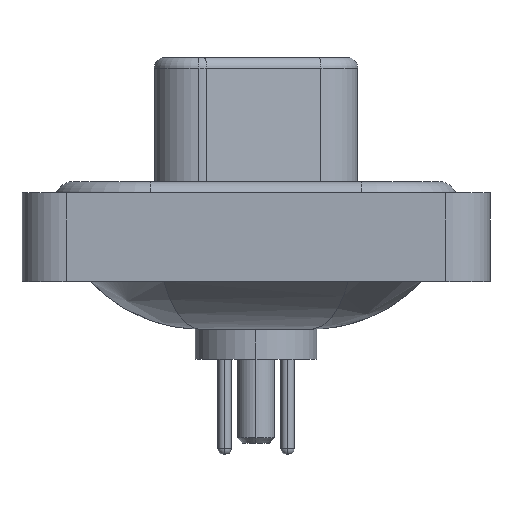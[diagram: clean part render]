
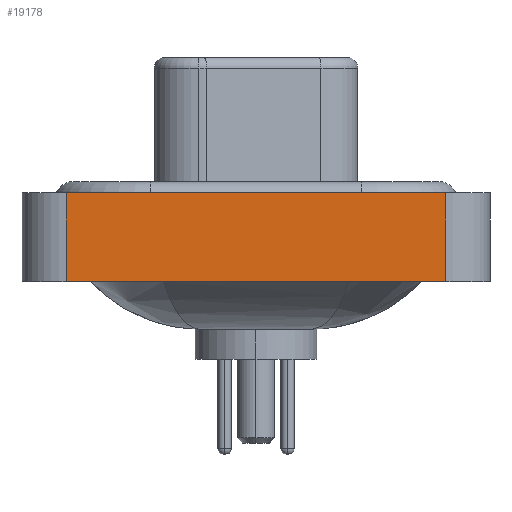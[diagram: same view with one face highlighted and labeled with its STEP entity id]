
A CAD part, left-side view. The second image highlights one B-rep face of the part: STEP entity #19178.
In plain terms, the highlighted planar face has unit normal (-1, 0, 0).
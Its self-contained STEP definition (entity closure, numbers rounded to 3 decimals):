
#711 = EDGE_LOOP ( 'NONE', ( #2815, #13599, #16392, #7864 ) ) ;
#886 = VECTOR ( 'NONE', #18986, 1000. ) ;
#1263 = DIRECTION ( 'NONE',  ( 0., 0., 1. ) ) ;
#2015 = VERTEX_POINT ( 'NONE', #18123 ) ;
#2815 = ORIENTED_EDGE ( 'NONE', *, *, #9867, .T. ) ;
#3252 = CARTESIAN_POINT ( 'NONE',  ( -7.3, -8.55, -3.6 ) ) ;
#3781 = VECTOR ( 'NONE', #5715, 1000. ) ;
#4097 = CARTESIAN_POINT ( 'NONE',  ( -7.3, 8.55, 0.4 ) ) ;
#4181 = AXIS2_PLACEMENT_3D ( 'NONE', #11735, #5859, #1263 ) ;
#5520 = LINE ( 'NONE', #7403, #3781 ) ;
#5615 = VERTEX_POINT ( 'NONE', #4097 ) ;
#5715 = DIRECTION ( 'NONE',  ( 0., -1., 0. ) ) ;
#5859 = DIRECTION ( 'NONE',  ( -1., 0., 0. ) ) ;
#6886 = DIRECTION ( 'NONE',  ( 0., 0., 1. ) ) ;
#7403 = CARTESIAN_POINT ( 'NONE',  ( -7.3, -8.55, -3.6 ) ) ;
#7864 = ORIENTED_EDGE ( 'NONE', *, *, #18214, .T. ) ;
#8739 = VERTEX_POINT ( 'NONE', #3252 ) ;
#8844 = DIRECTION ( 'NONE',  ( 0., -1., 0. ) ) ;
#8994 = EDGE_CURVE ( 'NONE', #5615, #10497, #10243, .T. ) ;
#9867 = EDGE_CURVE ( 'NONE', #8739, #10497, #14450, .T. ) ;
#10243 = LINE ( 'NONE', #10334, #18888 ) ;
#10334 = CARTESIAN_POINT ( 'NONE',  ( -7.3, -8.55, 0.4 ) ) ;
#10497 = VERTEX_POINT ( 'NONE', #16201 ) ;
#11261 = CARTESIAN_POINT ( 'NONE',  ( -7.3, 8.55, -3.6 ) ) ;
#11487 = CARTESIAN_POINT ( 'NONE',  ( -7.3, -8.55, -3.6 ) ) ;
#11735 = CARTESIAN_POINT ( 'NONE',  ( -7.3, -8.55, -3.6 ) ) ;
#13224 = PLANE ( 'NONE',  #4181 ) ;
#13599 = ORIENTED_EDGE ( 'NONE', *, *, #8994, .F. ) ;
#14450 = LINE ( 'NONE', #11487, #886 ) ;
#14613 = FACE_OUTER_BOUND ( 'NONE', #711, .T. ) ;
#15895 = LINE ( 'NONE', #11261, #16385 ) ;
#16201 = CARTESIAN_POINT ( 'NONE',  ( -7.3, -8.55, 0.4 ) ) ;
#16385 = VECTOR ( 'NONE', #6886, 1000. ) ;
#16392 = ORIENTED_EDGE ( 'NONE', *, *, #18543, .F. ) ;
#18123 = CARTESIAN_POINT ( 'NONE',  ( -7.3, 8.55, -3.6 ) ) ;
#18214 = EDGE_CURVE ( 'NONE', #2015, #8739, #5520, .T. ) ;
#18543 = EDGE_CURVE ( 'NONE', #2015, #5615, #15895, .T. ) ;
#18888 = VECTOR ( 'NONE', #8844, 1000. ) ;
#18986 = DIRECTION ( 'NONE',  ( 0., 0., 1. ) ) ;
#19178 = ADVANCED_FACE ( 'NONE', ( #14613 ), #13224, .T. ) ;
